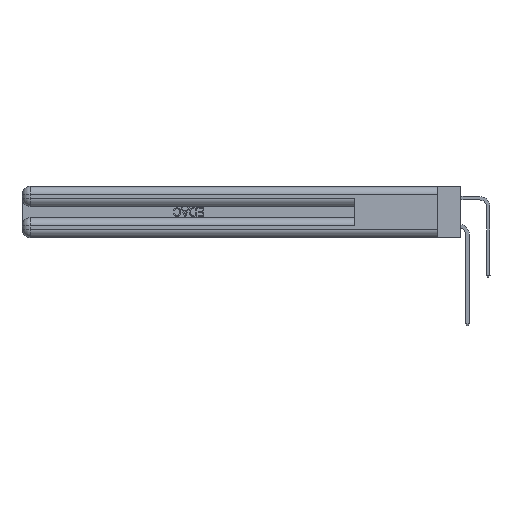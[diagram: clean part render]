
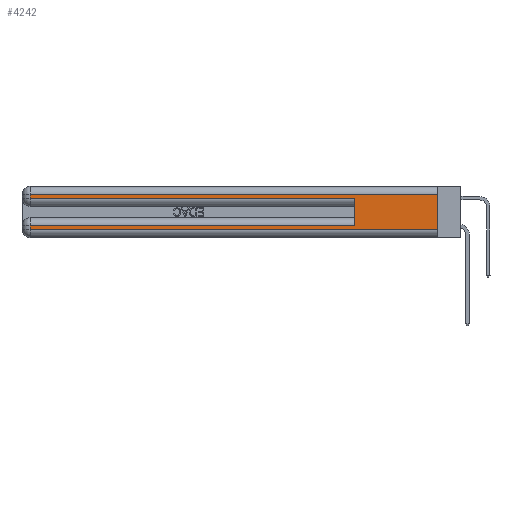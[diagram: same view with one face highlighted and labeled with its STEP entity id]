
A CAD part, left-side view. The second image highlights one B-rep face of the part: STEP entity #4242.
In plain terms, the highlighted planar face has unit normal (-1, 0, 0).
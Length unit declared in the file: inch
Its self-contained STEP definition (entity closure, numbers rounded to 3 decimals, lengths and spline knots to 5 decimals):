
#982 = CARTESIAN_POINT ( 'NONE',  ( 0., 2.94, 0.085 ) ) ;
#1565 = CARTESIAN_POINT ( 'NONE',  ( 0., 0., 0.37 ) ) ;
#3134 = VERTEX_POINT ( 'NONE', #38767 ) ;
#3425 = VECTOR ( 'NONE', #44171, 39.37008 ) ;
#3440 = VERTEX_POINT ( 'NONE', #982 ) ;
#3670 = ORIENTED_EDGE ( 'NONE', *, *, #35827, .T. ) ;
#4242 = ADVANCED_FACE ( 'NONE', ( #17774 ), #37739, .F. ) ;
#4561 = ORIENTED_EDGE ( 'NONE', *, *, #7950, .F. ) ;
#5229 = VECTOR ( 'NONE', #5305, 39.37008 ) ;
#5305 = DIRECTION ( 'NONE',  ( 0., 0., -1. ) ) ;
#6006 = CARTESIAN_POINT ( 'NONE',  ( 0., 0.6, 0.085 ) ) ;
#6196 = EDGE_CURVE ( 'NONE', #16354, #3440, #42591, .T. ) ;
#7950 = EDGE_CURVE ( 'NONE', #16354, #25978, #32021, .T. ) ;
#8822 = ORIENTED_EDGE ( 'NONE', *, *, #33853, .F. ) ;
#9032 = LINE ( 'NONE', #19634, #26890 ) ;
#9653 = LINE ( 'NONE', #33632, #27498 ) ;
#9674 = EDGE_CURVE ( 'NONE', #45138, #25978, #9032, .T. ) ;
#11474 = CARTESIAN_POINT ( 'NONE',  ( 0., 2.94, 0.37 ) ) ;
#11534 = LINE ( 'NONE', #40897, #28232 ) ;
#11850 = VERTEX_POINT ( 'NONE', #23583 ) ;
#12038 = VECTOR ( 'NONE', #25688, 39.37008 ) ;
#12466 = EDGE_CURVE ( 'NONE', #27409, #24460, #11534, .T. ) ;
#14158 = EDGE_CURVE ( 'NONE', #3440, #27409, #25319, .T. ) ;
#14532 = ORIENTED_EDGE ( 'NONE', *, *, #9674, .T. ) ;
#15427 = ORIENTED_EDGE ( 'NONE', *, *, #6196, .T. ) ;
#15593 = CARTESIAN_POINT ( 'NONE',  ( 0., 0.6, 0.145 ) ) ;
#16354 = VERTEX_POINT ( 'NONE', #6006 ) ;
#17686 = EDGE_LOOP ( 'NONE', ( #8822, #37403, #3670, #14532, #4561, #15427, #23526, #28159 ) ) ;
#17774 = FACE_OUTER_BOUND ( 'NONE', #17686, .T. ) ;
#19357 = CARTESIAN_POINT ( 'NONE',  ( 0., 0., 0.085 ) ) ;
#19634 = CARTESIAN_POINT ( 'NONE',  ( 0., 0., 0.285 ) ) ;
#20085 = CARTESIAN_POINT ( 'NONE',  ( 0., 0., 0.37 ) ) ;
#23224 = DIRECTION ( 'NONE',  ( 0., -1., 0. ) ) ;
#23526 = ORIENTED_EDGE ( 'NONE', *, *, #14158, .T. ) ;
#23583 = CARTESIAN_POINT ( 'NONE',  ( 0., 0., 0.31 ) ) ;
#23660 = DIRECTION ( 'NONE',  ( 0., 0., -1. ) ) ;
#24206 = VECTOR ( 'NONE', #46063, 39.37008 ) ;
#24460 = VERTEX_POINT ( 'NONE', #29359 ) ;
#25319 = LINE ( 'NONE', #42464, #24206 ) ;
#25688 = DIRECTION ( 'NONE',  ( 0., 0., 1. ) ) ;
#25978 = VERTEX_POINT ( 'NONE', #41810 ) ;
#26040 = CARTESIAN_POINT ( 'NONE',  ( 0., 2.94, 0.06 ) ) ;
#26890 = VECTOR ( 'NONE', #23224, 39.37008 ) ;
#27409 = VERTEX_POINT ( 'NONE', #26040 ) ;
#27498 = VECTOR ( 'NONE', #37193, 39.37008 ) ;
#28159 = ORIENTED_EDGE ( 'NONE', *, *, #12466, .T. ) ;
#28232 = VECTOR ( 'NONE', #37294, 39.37008 ) ;
#28910 = AXIS2_PLACEMENT_3D ( 'NONE', #20085, #44911, #23660 ) ;
#29359 = CARTESIAN_POINT ( 'NONE',  ( 0., 0., 0.06 ) ) ;
#30203 = LINE ( 'NONE', #11474, #45801 ) ;
#32021 = LINE ( 'NONE', #15593, #12038 ) ;
#32750 = DIRECTION ( 'NONE',  ( 0., 0., -1. ) ) ;
#33632 = CARTESIAN_POINT ( 'NONE',  ( 0., 0., 0.31 ) ) ;
#33853 = EDGE_CURVE ( 'NONE', #11850, #24460, #43186, .T. ) ;
#34519 = CARTESIAN_POINT ( 'NONE',  ( 0., 2.94, 0.285 ) ) ;
#35172 = EDGE_CURVE ( 'NONE', #11850, #3134, #9653, .T. ) ;
#35827 = EDGE_CURVE ( 'NONE', #3134, #45138, #30203, .T. ) ;
#37193 = DIRECTION ( 'NONE',  ( 0., 1., 0. ) ) ;
#37294 = DIRECTION ( 'NONE',  ( 0., -1., 0. ) ) ;
#37403 = ORIENTED_EDGE ( 'NONE', *, *, #35172, .T. ) ;
#37739 = PLANE ( 'NONE',  #28910 ) ;
#38767 = CARTESIAN_POINT ( 'NONE',  ( 0., 2.94, 0.31 ) ) ;
#40897 = CARTESIAN_POINT ( 'NONE',  ( 0., 0., 0.06 ) ) ;
#41810 = CARTESIAN_POINT ( 'NONE',  ( 0., 0.6, 0.285 ) ) ;
#42464 = CARTESIAN_POINT ( 'NONE',  ( 0., 2.94, 0.37 ) ) ;
#42591 = LINE ( 'NONE', #19357, #3425 ) ;
#43186 = LINE ( 'NONE', #1565, #5229 ) ;
#44171 = DIRECTION ( 'NONE',  ( 0., 1., 0. ) ) ;
#44911 = DIRECTION ( 'NONE',  ( 1., 0., 0. ) ) ;
#45138 = VERTEX_POINT ( 'NONE', #34519 ) ;
#45801 = VECTOR ( 'NONE', #32750, 39.37008 ) ;
#46063 = DIRECTION ( 'NONE',  ( 0., 0., -1. ) ) ;
